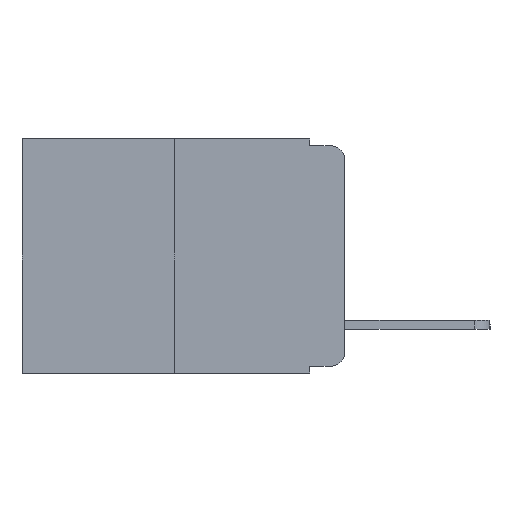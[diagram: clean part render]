
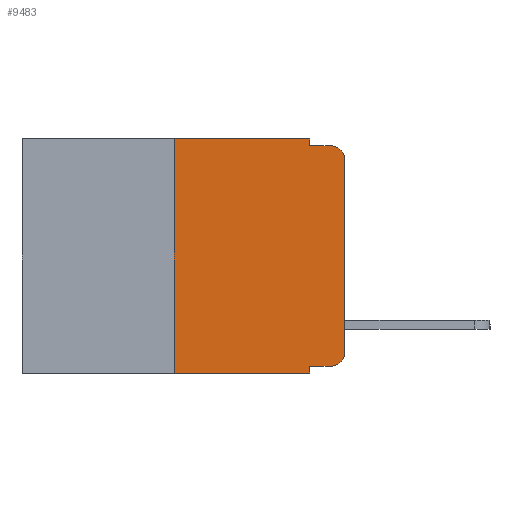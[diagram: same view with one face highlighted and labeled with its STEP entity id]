
A CAD part, left-side view. The second image highlights one B-rep face of the part: STEP entity #9483.
In plain terms, the highlighted planar face has unit normal (-1, 0, 0).
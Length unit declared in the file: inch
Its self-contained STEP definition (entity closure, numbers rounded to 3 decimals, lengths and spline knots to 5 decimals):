
#15 = PLANE ( 'NONE',  #10576 ) ;
#30 = ORIENTED_EDGE ( 'NONE', *, *, #14861, .F. ) ;
#346 = ORIENTED_EDGE ( 'NONE', *, *, #10460, .F. ) ;
#707 = DIRECTION ( 'NONE',  ( 0., 0., -1. ) ) ;
#794 = CARTESIAN_POINT ( 'NONE',  ( 0., 0., -0.313 ) ) ;
#1374 = VERTEX_POINT ( 'NONE', #3794 ) ;
#1402 = DIRECTION ( 'NONE',  ( 0., 0., -1. ) ) ;
#1736 = VERTEX_POINT ( 'NONE', #15318 ) ;
#2023 = CARTESIAN_POINT ( 'NONE',  ( 0., 0.25, 0. ) ) ;
#2095 = VECTOR ( 'NONE', #14652, 39.37008 ) ;
#2175 = CARTESIAN_POINT ( 'NONE',  ( 0., 0.473, 0. ) ) ;
#2431 = FACE_OUTER_BOUND ( 'NONE', #11295, .T. ) ;
#2742 = DIRECTION ( 'NONE',  ( 0., 0., 1. ) ) ;
#2786 = CIRCLE ( 'NONE', #4827, 0.02 ) ;
#2827 = CIRCLE ( 'NONE', #8969, 0.02 ) ;
#2941 = DIRECTION ( 'NONE',  ( -1., 0., 0. ) ) ;
#3170 = CARTESIAN_POINT ( 'NONE',  ( 0., 0.051, -0.333 ) ) ;
#3241 = CARTESIAN_POINT ( 'NONE',  ( 0., 0.051, -0.343 ) ) ;
#3553 = CARTESIAN_POINT ( 'NONE',  ( 0., 0.25, -0.343 ) ) ;
#3794 = CARTESIAN_POINT ( 'NONE',  ( 0., 0.051, -0.01 ) ) ;
#3944 = LINE ( 'NONE', #12510, #6874 ) ;
#4063 = EDGE_CURVE ( 'NONE', #5486, #11782, #8705, .T. ) ;
#4383 = EDGE_CURVE ( 'NONE', #7872, #1374, #4444, .T. ) ;
#4444 = LINE ( 'NONE', #9324, #12344 ) ;
#4738 = VECTOR ( 'NONE', #14960, 39.37008 ) ;
#4827 = AXIS2_PLACEMENT_3D ( 'NONE', #13922, #2941, #707 ) ;
#5172 = DIRECTION ( 'NONE',  ( 0., -1., 0. ) ) ;
#5234 = DIRECTION ( 'NONE',  ( 1., 0., 0. ) ) ;
#5486 = VERTEX_POINT ( 'NONE', #3170 ) ;
#5617 = ORIENTED_EDGE ( 'NONE', *, *, #10635, .T. ) ;
#5941 = DIRECTION ( 'NONE',  ( 0., -1., 0. ) ) ;
#6119 = CARTESIAN_POINT ( 'NONE',  ( 0., 0.02, -0.313 ) ) ;
#6125 = EDGE_CURVE ( 'NONE', #14196, #12626, #2827, .T. ) ;
#6148 = CARTESIAN_POINT ( 'NONE',  ( 0., 0.051, 0. ) ) ;
#6316 = LINE ( 'NONE', #11168, #4738 ) ;
#6537 = VECTOR ( 'NONE', #13324, 39.37008 ) ;
#6835 = EDGE_CURVE ( 'NONE', #9160, #7872, #10964, .T. ) ;
#6874 = VECTOR ( 'NONE', #2742, 39.37008 ) ;
#6918 = DIRECTION ( 'NONE',  ( 0., 0., 1. ) ) ;
#7641 = CARTESIAN_POINT ( 'NONE',  ( 0., 0.25, 0. ) ) ;
#7872 = VERTEX_POINT ( 'NONE', #6148 ) ;
#8380 = ORIENTED_EDGE ( 'NONE', *, *, #4383, .F. ) ;
#8672 = ORIENTED_EDGE ( 'NONE', *, *, #6835, .F. ) ;
#8690 = VECTOR ( 'NONE', #5941, 39.37008 ) ;
#8705 = LINE ( 'NONE', #10862, #2095 ) ;
#8755 = CARTESIAN_POINT ( 'NONE',  ( 0., 0.473, 0. ) ) ;
#8779 = CARTESIAN_POINT ( 'NONE',  ( 0., 0.051, -0.333 ) ) ;
#8969 = AXIS2_PLACEMENT_3D ( 'NONE', #6119, #14699, #12096 ) ;
#9105 = ORIENTED_EDGE ( 'NONE', *, *, #6125, .T. ) ;
#9141 = LINE ( 'NONE', #2023, #11113 ) ;
#9160 = VERTEX_POINT ( 'NONE', #7641 ) ;
#9324 = CARTESIAN_POINT ( 'NONE',  ( 0., 0.051, 0. ) ) ;
#9451 = VERTEX_POINT ( 'NONE', #3553 ) ;
#9483 = ADVANCED_FACE ( 'NONE', ( #2431 ), #15, .F. ) ;
#10460 = EDGE_CURVE ( 'NONE', #1374, #11665, #6316, .T. ) ;
#10576 = AXIS2_PLACEMENT_3D ( 'NONE', #8755, #5234, #1402 ) ;
#10635 = EDGE_CURVE ( 'NONE', #9451, #11782, #13401, .T. ) ;
#10862 = CARTESIAN_POINT ( 'NONE',  ( 0., 0.051, 0. ) ) ;
#10964 = LINE ( 'NONE', #2175, #8690 ) ;
#11113 = VECTOR ( 'NONE', #6918, 39.37008 ) ;
#11168 = CARTESIAN_POINT ( 'NONE',  ( 0., 0.051, -0.01 ) ) ;
#11295 = EDGE_LOOP ( 'NONE', ( #11499, #15279, #346, #8380, #8672, #30, #5617, #15408, #14902, #9105 ) ) ;
#11499 = ORIENTED_EDGE ( 'NONE', *, *, #13798, .T. ) ;
#11615 = EDGE_CURVE ( 'NONE', #5486, #14196, #12539, .T. ) ;
#11665 = VERTEX_POINT ( 'NONE', #14962 ) ;
#11782 = VERTEX_POINT ( 'NONE', #3241 ) ;
#11871 = CARTESIAN_POINT ( 'NONE',  ( 0., 0.473, -0.343 ) ) ;
#12096 = DIRECTION ( 'NONE',  ( 0., 0., -1. ) ) ;
#12344 = VECTOR ( 'NONE', #14232, 39.37008 ) ;
#12475 = EDGE_CURVE ( 'NONE', #1736, #11665, #2786, .T. ) ;
#12510 = CARTESIAN_POINT ( 'NONE',  ( 0., 0., 0. ) ) ;
#12539 = LINE ( 'NONE', #8779, #13026 ) ;
#12626 = VERTEX_POINT ( 'NONE', #794 ) ;
#13026 = VECTOR ( 'NONE', #5172, 39.37008 ) ;
#13324 = DIRECTION ( 'NONE',  ( 0., -1., 0. ) ) ;
#13401 = LINE ( 'NONE', #11871, #6537 ) ;
#13798 = EDGE_CURVE ( 'NONE', #12626, #1736, #3944, .T. ) ;
#13922 = CARTESIAN_POINT ( 'NONE',  ( 0., 0.02, -0.03 ) ) ;
#14196 = VERTEX_POINT ( 'NONE', #15667 ) ;
#14232 = DIRECTION ( 'NONE',  ( 0., 0., -1. ) ) ;
#14652 = DIRECTION ( 'NONE',  ( 0., 0., -1. ) ) ;
#14699 = DIRECTION ( 'NONE',  ( -1., 0., 0. ) ) ;
#14861 = EDGE_CURVE ( 'NONE', #9451, #9160, #9141, .T. ) ;
#14902 = ORIENTED_EDGE ( 'NONE', *, *, #11615, .T. ) ;
#14960 = DIRECTION ( 'NONE',  ( 0., -1., 0. ) ) ;
#14962 = CARTESIAN_POINT ( 'NONE',  ( 0., 0.02, -0.01 ) ) ;
#15279 = ORIENTED_EDGE ( 'NONE', *, *, #12475, .T. ) ;
#15318 = CARTESIAN_POINT ( 'NONE',  ( 0., 0., -0.03 ) ) ;
#15408 = ORIENTED_EDGE ( 'NONE', *, *, #4063, .F. ) ;
#15667 = CARTESIAN_POINT ( 'NONE',  ( 0., 0.02, -0.333 ) ) ;
